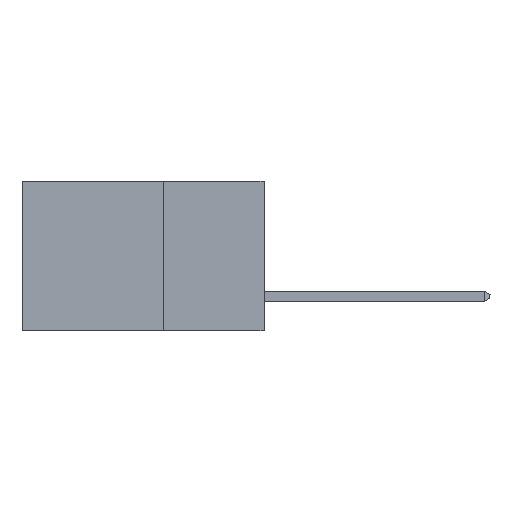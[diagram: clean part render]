
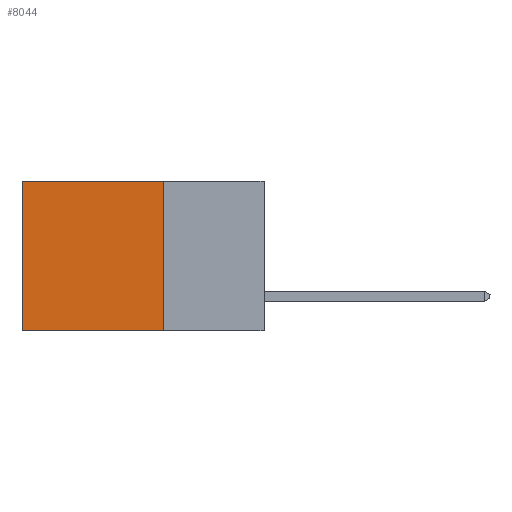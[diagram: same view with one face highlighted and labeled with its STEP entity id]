
A CAD part, left-side view. The second image highlights one B-rep face of the part: STEP entity #8044.
In plain terms, the highlighted planar face has unit normal (-1, 0, 0).
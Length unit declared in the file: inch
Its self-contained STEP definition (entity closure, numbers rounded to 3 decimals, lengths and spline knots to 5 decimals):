
#252 = LINE ( 'NONE', #7388, #3606 ) ;
#982 = CARTESIAN_POINT ( 'NONE',  ( 0.2615, 0.25, -0.37 ) ) ;
#1253 = CARTESIAN_POINT ( 'NONE',  ( 0.2615, 0.25, -0.37 ) ) ;
#1922 = AXIS2_PLACEMENT_3D ( 'NONE', #8111, #2023, #11767 ) ;
#2023 = DIRECTION ( 'NONE',  ( 1., 0., 0. ) ) ;
#2689 = EDGE_CURVE ( 'NONE', #9862, #3520, #7305, .T. ) ;
#3520 = VERTEX_POINT ( 'NONE', #3813 ) ;
#3606 = VECTOR ( 'NONE', #12256, 39.37008 ) ;
#3615 = ORIENTED_EDGE ( 'NONE', *, *, #14690, .T. ) ;
#3813 = CARTESIAN_POINT ( 'NONE',  ( 0.2615, 0.6, 0. ) ) ;
#4665 = CARTESIAN_POINT ( 'NONE',  ( 0.2615, 0.6, -0.37 ) ) ;
#5587 = VERTEX_POINT ( 'NONE', #982 ) ;
#7141 = FACE_OUTER_BOUND ( 'NONE', #8644, .T. ) ;
#7305 = LINE ( 'NONE', #8827, #13174 ) ;
#7388 = CARTESIAN_POINT ( 'NONE',  ( 0.2615, 0.25, -0.37 ) ) ;
#7421 = ORIENTED_EDGE ( 'NONE', *, *, #10268, .F. ) ;
#8044 = ADVANCED_FACE ( 'NONE', ( #7141 ), #15295, .F. ) ;
#8111 = CARTESIAN_POINT ( 'NONE',  ( 0.2615, 0.25, -0.37 ) ) ;
#8552 = DIRECTION ( 'NONE',  ( 0., 0., -1. ) ) ;
#8644 = EDGE_LOOP ( 'NONE', ( #3615, #13458, #7421, #13092 ) ) ;
#8827 = CARTESIAN_POINT ( 'NONE',  ( 0.2615, 0.25, 0. ) ) ;
#9475 = DIRECTION ( 'NONE',  ( 0., 0., -1. ) ) ;
#9698 = VERTEX_POINT ( 'NONE', #14398 ) ;
#9862 = VERTEX_POINT ( 'NONE', #13356 ) ;
#10268 = EDGE_CURVE ( 'NONE', #9862, #5587, #13491, .T. ) ;
#11767 = DIRECTION ( 'NONE',  ( 0., 0., -1. ) ) ;
#11871 = LINE ( 'NONE', #4665, #15174 ) ;
#11998 = EDGE_CURVE ( 'NONE', #5587, #9698, #252, .T. ) ;
#12252 = VECTOR ( 'NONE', #8552, 39.37008 ) ;
#12256 = DIRECTION ( 'NONE',  ( 0., 1., 0. ) ) ;
#13092 = ORIENTED_EDGE ( 'NONE', *, *, #2689, .T. ) ;
#13174 = VECTOR ( 'NONE', #13688, 39.37008 ) ;
#13356 = CARTESIAN_POINT ( 'NONE',  ( 0.2615, 0.25, 0. ) ) ;
#13458 = ORIENTED_EDGE ( 'NONE', *, *, #11998, .F. ) ;
#13491 = LINE ( 'NONE', #1253, #12252 ) ;
#13688 = DIRECTION ( 'NONE',  ( 0., 1., 0. ) ) ;
#14398 = CARTESIAN_POINT ( 'NONE',  ( 0.2615, 0.6, -0.37 ) ) ;
#14690 = EDGE_CURVE ( 'NONE', #3520, #9698, #11871, .T. ) ;
#15174 = VECTOR ( 'NONE', #9475, 39.37008 ) ;
#15295 = PLANE ( 'NONE',  #1922 ) ;
